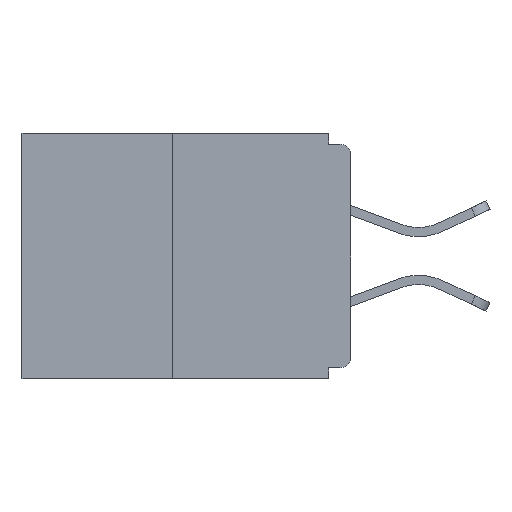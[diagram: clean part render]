
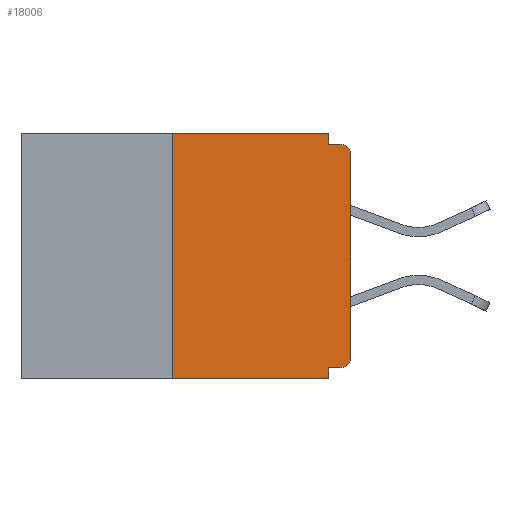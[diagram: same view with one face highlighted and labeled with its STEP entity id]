
A CAD part, left-side view. The second image highlights one B-rep face of the part: STEP entity #18006.
In plain terms, the highlighted planar face has unit normal (-1, 0, 0).
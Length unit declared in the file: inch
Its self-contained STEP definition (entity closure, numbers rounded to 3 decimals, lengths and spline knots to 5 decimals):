
#218 = VECTOR ( 'NONE', #1844, 39.37008 ) ;
#534 = CARTESIAN_POINT ( 'NONE',  ( 0., 0.46, 0. ) ) ;
#927 = LINE ( 'NONE', #534, #12292 ) ;
#1579 = AXIS2_PLACEMENT_3D ( 'NONE', #5340, #12742, #3955 ) ;
#1734 = VECTOR ( 'NONE', #9696, 39.37008 ) ;
#1844 = DIRECTION ( 'NONE',  ( 0., 0., 1. ) ) ;
#2138 = ORIENTED_EDGE ( 'NONE', *, *, #11551, .F. ) ;
#2202 = LINE ( 'NONE', #6608, #1734 ) ;
#2542 = CARTESIAN_POINT ( 'NONE',  ( 0., 0.031, 0. ) ) ;
#3137 = VERTEX_POINT ( 'NONE', #9171 ) ;
#3441 = VERTEX_POINT ( 'NONE', #18896 ) ;
#3489 = EDGE_CURVE ( 'NONE', #18387, #16764, #5537, .T. ) ;
#3552 = VECTOR ( 'NONE', #13435, 39.37008 ) ;
#3629 = CARTESIAN_POINT ( 'NONE',  ( 0., 0.031, -0.015 ) ) ;
#3713 = CIRCLE ( 'NONE', #1579, 0.015 ) ;
#3746 = AXIS2_PLACEMENT_3D ( 'NONE', #12679, #6627, #11289 ) ;
#3776 = DIRECTION ( 'NONE',  ( -1., 0., 0. ) ) ;
#3955 = DIRECTION ( 'NONE',  ( 0., 0., -1. ) ) ;
#3971 = VERTEX_POINT ( 'NONE', #13171 ) ;
#4088 = ORIENTED_EDGE ( 'NONE', *, *, #14977, .T. ) ;
#4371 = ORIENTED_EDGE ( 'NONE', *, *, #12809, .F. ) ;
#4524 = VECTOR ( 'NONE', #7086, 39.37008 ) ;
#4840 = CARTESIAN_POINT ( 'NONE',  ( 0., 0.031, 0. ) ) ;
#5316 = DIRECTION ( 'NONE',  ( 0., 0., -1. ) ) ;
#5340 = CARTESIAN_POINT ( 'NONE',  ( 0., 0.015, -0.03 ) ) ;
#5344 = EDGE_CURVE ( 'NONE', #7947, #3137, #17779, .T. ) ;
#5537 = CIRCLE ( 'NONE', #13344, 0.015 ) ;
#5832 = EDGE_CURVE ( 'NONE', #8354, #11036, #9086, .T. ) ;
#5976 = LINE ( 'NONE', #11890, #3552 ) ;
#6550 = DIRECTION ( 'NONE',  ( 0., 0., 1. ) ) ;
#6608 = CARTESIAN_POINT ( 'NONE',  ( 0., 0., -0.328 ) ) ;
#6627 = DIRECTION ( 'NONE',  ( 1., 0., 0. ) ) ;
#6687 = CARTESIAN_POINT ( 'NONE',  ( 0., 0., 0. ) ) ;
#7086 = DIRECTION ( 'NONE',  ( 0., 0., -1. ) ) ;
#7296 = CARTESIAN_POINT ( 'NONE',  ( 0., 0.031, -0.328 ) ) ;
#7947 = VERTEX_POINT ( 'NONE', #7296 ) ;
#8099 = DIRECTION ( 'NONE',  ( 0., -1., 0. ) ) ;
#8261 = CARTESIAN_POINT ( 'NONE',  ( 0., 0.015, -0.313 ) ) ;
#8354 = VERTEX_POINT ( 'NONE', #4840 ) ;
#8410 = EDGE_CURVE ( 'NONE', #16764, #18915, #19655, .T. ) ;
#9086 = LINE ( 'NONE', #2542, #4524 ) ;
#9171 = CARTESIAN_POINT ( 'NONE',  ( 0., 0.031, -0.343 ) ) ;
#9349 = LINE ( 'NONE', #10993, #218 ) ;
#9551 = VECTOR ( 'NONE', #13733, 39.37008 ) ;
#9696 = DIRECTION ( 'NONE',  ( 0., 1., 0. ) ) ;
#10087 = ORIENTED_EDGE ( 'NONE', *, *, #5344, .F. ) ;
#10180 = CARTESIAN_POINT ( 'NONE',  ( 0., 0.25, -0.343 ) ) ;
#10192 = CARTESIAN_POINT ( 'NONE',  ( 0., 0., -0.313 ) ) ;
#10348 = ORIENTED_EDGE ( 'NONE', *, *, #8410, .T. ) ;
#10760 = ORIENTED_EDGE ( 'NONE', *, *, #5832, .F. ) ;
#10993 = CARTESIAN_POINT ( 'NONE',  ( 0., 0.25, 0. ) ) ;
#11036 = VERTEX_POINT ( 'NONE', #3629 ) ;
#11289 = DIRECTION ( 'NONE',  ( 0., 0., -1. ) ) ;
#11551 = EDGE_CURVE ( 'NONE', #11036, #3971, #13221, .T. ) ;
#11838 = EDGE_CURVE ( 'NONE', #18915, #3971, #3713, .T. ) ;
#11890 = CARTESIAN_POINT ( 'NONE',  ( 0., 0.46, -0.343 ) ) ;
#12292 = VECTOR ( 'NONE', #18957, 39.37008 ) ;
#12642 = VERTEX_POINT ( 'NONE', #10180 ) ;
#12679 = CARTESIAN_POINT ( 'NONE',  ( 0., 0.46, 0. ) ) ;
#12742 = DIRECTION ( 'NONE',  ( -1., 0., 0. ) ) ;
#12809 = EDGE_CURVE ( 'NONE', #18387, #7947, #2202, .T. ) ;
#12873 = ORIENTED_EDGE ( 'NONE', *, *, #14306, .F. ) ;
#12916 = PLANE ( 'NONE',  #3746 ) ;
#13034 = ORIENTED_EDGE ( 'NONE', *, *, #18217, .F. ) ;
#13171 = CARTESIAN_POINT ( 'NONE',  ( 0., 0.015, -0.015 ) ) ;
#13221 = LINE ( 'NONE', #18816, #15435 ) ;
#13344 = AXIS2_PLACEMENT_3D ( 'NONE', #8261, #3776, #5316 ) ;
#13435 = DIRECTION ( 'NONE',  ( 0., -1., 0. ) ) ;
#13504 = EDGE_LOOP ( 'NONE', ( #13034, #12873, #4088, #10087, #4371, #14264, #10348, #19503, #2138, #10760 ) ) ;
#13733 = DIRECTION ( 'NONE',  ( 0., 0., -1. ) ) ;
#14264 = ORIENTED_EDGE ( 'NONE', *, *, #3489, .T. ) ;
#14306 = EDGE_CURVE ( 'NONE', #12642, #3441, #9349, .T. ) ;
#14624 = CARTESIAN_POINT ( 'NONE',  ( 0., 0.015, -0.328 ) ) ;
#14977 = EDGE_CURVE ( 'NONE', #12642, #3137, #5976, .T. ) ;
#15228 = CARTESIAN_POINT ( 'NONE',  ( 0., 0.031, -0.343 ) ) ;
#15435 = VECTOR ( 'NONE', #8099, 39.37008 ) ;
#16764 = VERTEX_POINT ( 'NONE', #10192 ) ;
#17595 = FACE_OUTER_BOUND ( 'NONE', #13504, .T. ) ;
#17779 = LINE ( 'NONE', #15228, #9551 ) ;
#18006 = ADVANCED_FACE ( 'NONE', ( #17595 ), #12916, .F. ) ;
#18217 = EDGE_CURVE ( 'NONE', #3441, #8354, #927, .T. ) ;
#18387 = VERTEX_POINT ( 'NONE', #14624 ) ;
#18690 = VECTOR ( 'NONE', #6550, 39.37008 ) ;
#18816 = CARTESIAN_POINT ( 'NONE',  ( 0., 0., -0.015 ) ) ;
#18896 = CARTESIAN_POINT ( 'NONE',  ( 0., 0.25, 0. ) ) ;
#18915 = VERTEX_POINT ( 'NONE', #19810 ) ;
#18957 = DIRECTION ( 'NONE',  ( 0., -1., 0. ) ) ;
#19503 = ORIENTED_EDGE ( 'NONE', *, *, #11838, .T. ) ;
#19655 = LINE ( 'NONE', #6687, #18690 ) ;
#19810 = CARTESIAN_POINT ( 'NONE',  ( 0., 0., -0.03 ) ) ;
